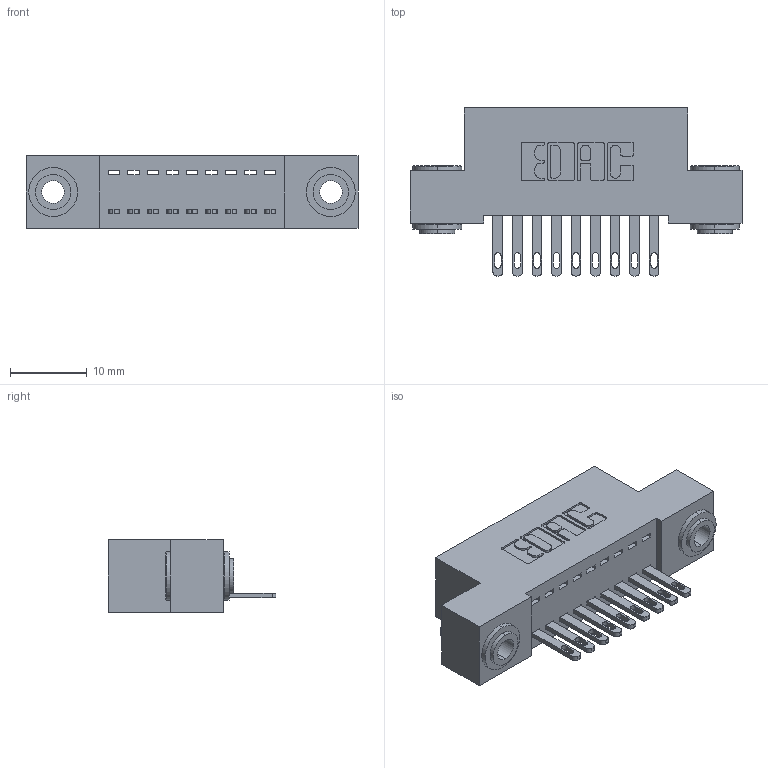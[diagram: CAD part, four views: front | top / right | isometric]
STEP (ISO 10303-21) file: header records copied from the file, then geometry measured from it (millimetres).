
FILE_DESCRIPTION (( 'STEP AP203' ), '1' );
FILE_NAME ('342-009-500-103.STEP', '2018-08-10T12:38:03', ( '' ), ( '' ), 'SwSTEP 2.0', 'SolidWorks 2016', '' );
FILE_SCHEMA (( 'CONFIG_CONTROL_DESIGN' ));
Length unit declared in the file: inch
Products named in the file (4): 342 Part_.156 TH; 345-292-001_345-293-100; 342-250-002_345-250-002-102; 342-009-500-103
Assembly tree (12 placements, depth 2):
  342-009-500-103
    342 Part_.156 TH
    345-292-001_345-293-100  x9
    342-250-002_345-250-002-102  x2
Bounding box: 43.18 x 21.85 x 9.4 mm (x, y, z)
Volume: 3692.9 mm3; surface area: 5050.5 mm2
Topology: 12 solids, 12 shells, 634 faces, 1887 edges, 1254 vertices
Faces by surface type: plane 400, cylinder 226, cone 8
Entity records: 10218 total; most frequent: CARTESIAN_POINT 1744, ORIENTED_EDGE 1682, DIRECTION 1573, EDGE_CURVE 841, LINE 685, VECTOR 685, VERTEX_POINT 558, AXIS2_PLACEMENT_3D 444
